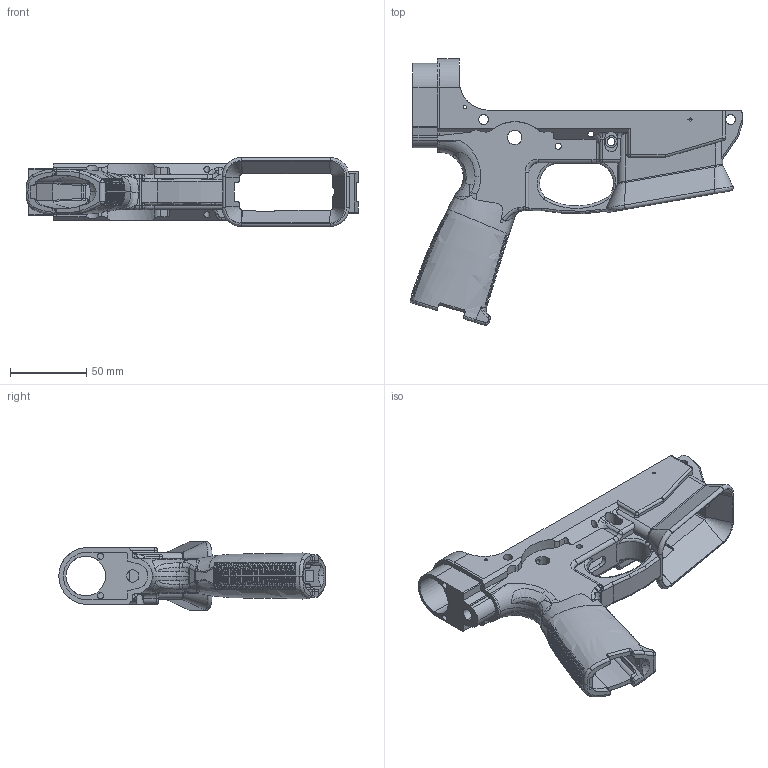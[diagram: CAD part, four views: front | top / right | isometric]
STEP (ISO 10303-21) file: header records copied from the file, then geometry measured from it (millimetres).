
FILE_DESCRIPTION (( 'STEP AP203' ), '1' );
FILE_NAME ('mbbi_monolithic__front.STEP', '2022-06-11T19:52:47', ( '' ), ( '' ), 'SwSTEP 2.0', 'SolidWorks 2021', '' );
FILE_SCHEMA (( 'CONFIG_CONTROL_DESIGN' ));
Length unit declared in the file: millimetre
Products named in the file (1): mbbi_monolithic__front
Bounding box: 217.56 x 174.49 x 45.01 mm (x, y, z)
Volume: 220305.8 mm3; surface area: 86263.2 mm2
Topology: 1 solids, 3 shells, 1225 faces, 3533 edges, 2289 vertices
Faces by surface type: plane 489, bspline 366, cylinder 299, torus 45, sphere 18, cone 8
Entity records: 85259 total; most frequent: CARTESIAN_POINT 57044, ORIENTED_EDGE 7024, DIRECTION 4266, EDGE_CURVE 3512, VERTEX_POINT 2289, B_SPLINE_CURVE_WITH_KNOTS 1535, AXIS2_PLACEMENT_3D 1525, EDGE_LOOP 1265
